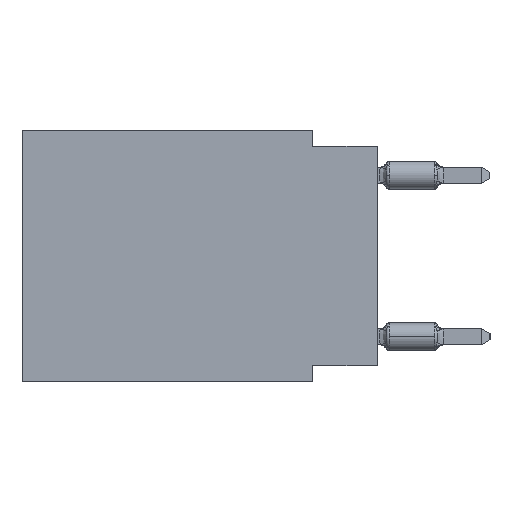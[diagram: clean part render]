
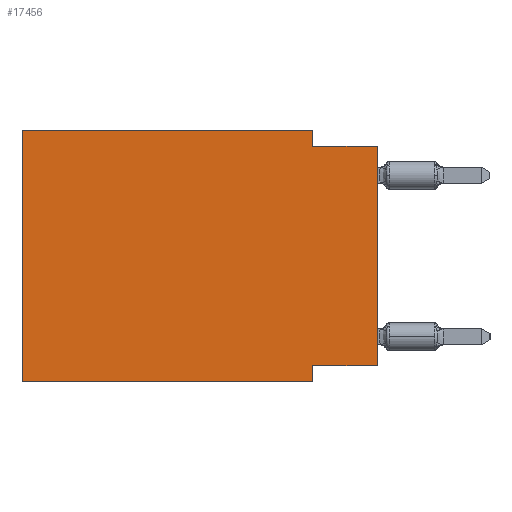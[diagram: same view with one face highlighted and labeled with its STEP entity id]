
A CAD part, left-side view. The second image highlights one B-rep face of the part: STEP entity #17456.
In plain terms, the highlighted planar face has unit normal (-1, 0, 0).
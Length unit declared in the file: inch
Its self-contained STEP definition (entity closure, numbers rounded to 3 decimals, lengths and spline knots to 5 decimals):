
#1050 = VERTEX_POINT ( 'NONE', #19948 ) ;
#2137 = CARTESIAN_POINT ( 'NONE',  ( 0., 0.1, 0. ) ) ;
#2324 = LINE ( 'NONE', #13500, #18718 ) ;
#3995 = VECTOR ( 'NONE', #16731, 39.37008 ) ;
#4267 = EDGE_CURVE ( 'NONE', #31240, #11778, #5981, .T. ) ;
#4664 = VECTOR ( 'NONE', #13489, 39.37008 ) ;
#4799 = LINE ( 'NONE', #8009, #45112 ) ;
#5981 = LINE ( 'NONE', #2137, #26511 ) ;
#6827 = ORIENTED_EDGE ( 'NONE', *, *, #16421, .T. ) ;
#6852 = LINE ( 'NONE', #17602, #4664 ) ;
#6977 = VERTEX_POINT ( 'NONE', #22000 ) ;
#7912 = ORIENTED_EDGE ( 'NONE', *, *, #27644, .F. ) ;
#8009 = CARTESIAN_POINT ( 'NONE',  ( 0., 0., -0.365 ) ) ;
#9197 = DIRECTION ( 'NONE',  ( 0., 0., 1. ) ) ;
#10527 = CARTESIAN_POINT ( 'NONE',  ( 0., 0., -0.025 ) ) ;
#10543 = VERTEX_POINT ( 'NONE', #11025 ) ;
#11025 = CARTESIAN_POINT ( 'NONE',  ( 0., 0.1, -0.39 ) ) ;
#11557 = CARTESIAN_POINT ( 'NONE',  ( 0., 0.55, 0. ) ) ;
#11778 = VERTEX_POINT ( 'NONE', #34912 ) ;
#13384 = ORIENTED_EDGE ( 'NONE', *, *, #4267, .F. ) ;
#13489 = DIRECTION ( 'NONE',  ( 0., 0., 1. ) ) ;
#13500 = CARTESIAN_POINT ( 'NONE',  ( 0., 0., 0. ) ) ;
#14973 = PLANE ( 'NONE',  #23759 ) ;
#16421 = EDGE_CURVE ( 'NONE', #6977, #10543, #27029, .T. ) ;
#16660 = CARTESIAN_POINT ( 'NONE',  ( 0., 0., -0.365 ) ) ;
#16731 = DIRECTION ( 'NONE',  ( 0., -1., 0. ) ) ;
#16822 = DIRECTION ( 'NONE',  ( 0., 0., -1. ) ) ;
#16897 = ORIENTED_EDGE ( 'NONE', *, *, #20534, .F. ) ;
#17456 = ADVANCED_FACE ( 'NONE', ( #18856 ), #14973, .F. ) ;
#17602 = CARTESIAN_POINT ( 'NONE',  ( 0., 0.55, 0. ) ) ;
#17748 = VECTOR ( 'NONE', #31151, 39.37008 ) ;
#18718 = VECTOR ( 'NONE', #9197, 39.37008 ) ;
#18856 = FACE_OUTER_BOUND ( 'NONE', #32960, .T. ) ;
#18990 = VECTOR ( 'NONE', #32976, 39.37008 ) ;
#19009 = CARTESIAN_POINT ( 'NONE',  ( 0., 0.55, 0. ) ) ;
#19614 = CARTESIAN_POINT ( 'NONE',  ( 0., 0.1, -0.39 ) ) ;
#19941 = DIRECTION ( 'NONE',  ( 0., 0., -1. ) ) ;
#19948 = CARTESIAN_POINT ( 'NONE',  ( 0., 0.1, -0.365 ) ) ;
#20534 = EDGE_CURVE ( 'NONE', #38801, #1050, #4799, .T. ) ;
#21630 = VERTEX_POINT ( 'NONE', #10527 ) ;
#22000 = CARTESIAN_POINT ( 'NONE',  ( 0., 0.55, -0.39 ) ) ;
#22059 = DIRECTION ( 'NONE',  ( 0., 0., -1. ) ) ;
#22994 = EDGE_CURVE ( 'NONE', #1050, #10543, #36786, .T. ) ;
#23759 = AXIS2_PLACEMENT_3D ( 'NONE', #11557, #40342, #22059 ) ;
#26177 = VECTOR ( 'NONE', #16822, 39.37008 ) ;
#26245 = CARTESIAN_POINT ( 'NONE',  ( 0., 0.1, 0. ) ) ;
#26406 = ORIENTED_EDGE ( 'NONE', *, *, #42410, .F. ) ;
#26511 = VECTOR ( 'NONE', #19941, 39.37008 ) ;
#27029 = LINE ( 'NONE', #34146, #3995 ) ;
#27644 = EDGE_CURVE ( 'NONE', #32630, #31240, #36424, .T. ) ;
#31151 = DIRECTION ( 'NONE',  ( 0., -1., 0. ) ) ;
#31240 = VERTEX_POINT ( 'NONE', #26245 ) ;
#31780 = ORIENTED_EDGE ( 'NONE', *, *, #22994, .F. ) ;
#32630 = VERTEX_POINT ( 'NONE', #40495 ) ;
#32960 = EDGE_LOOP ( 'NONE', ( #39267, #26406, #13384, #7912, #44277, #6827, #31780, #16897 ) ) ;
#32976 = DIRECTION ( 'NONE',  ( 0., -1., 0. ) ) ;
#34146 = CARTESIAN_POINT ( 'NONE',  ( 0., 0.55, -0.39 ) ) ;
#34212 = EDGE_CURVE ( 'NONE', #6977, #32630, #6852, .T. ) ;
#34912 = CARTESIAN_POINT ( 'NONE',  ( 0., 0.1, -0.025 ) ) ;
#36424 = LINE ( 'NONE', #19009, #18990 ) ;
#36545 = EDGE_CURVE ( 'NONE', #38801, #21630, #2324, .T. ) ;
#36786 = LINE ( 'NONE', #19614, #26177 ) ;
#38697 = CARTESIAN_POINT ( 'NONE',  ( 0., 0., -0.025 ) ) ;
#38801 = VERTEX_POINT ( 'NONE', #16660 ) ;
#38917 = LINE ( 'NONE', #38697, #17748 ) ;
#39267 = ORIENTED_EDGE ( 'NONE', *, *, #36545, .T. ) ;
#40342 = DIRECTION ( 'NONE',  ( 1., 0., 0. ) ) ;
#40495 = CARTESIAN_POINT ( 'NONE',  ( 0., 0.55, 0. ) ) ;
#42410 = EDGE_CURVE ( 'NONE', #11778, #21630, #38917, .T. ) ;
#42762 = DIRECTION ( 'NONE',  ( 0., 1., 0. ) ) ;
#44277 = ORIENTED_EDGE ( 'NONE', *, *, #34212, .F. ) ;
#45112 = VECTOR ( 'NONE', #42762, 39.37008 ) ;
